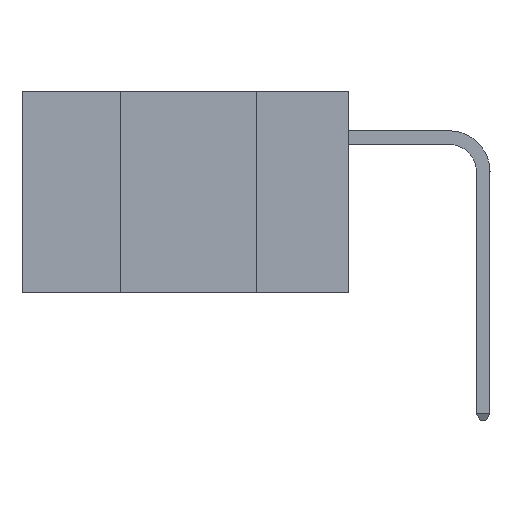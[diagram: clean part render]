
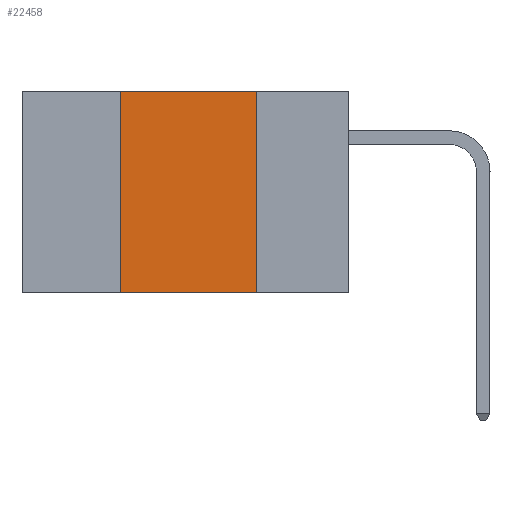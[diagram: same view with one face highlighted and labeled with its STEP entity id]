
A CAD part, left-side view. The second image highlights one B-rep face of the part: STEP entity #22458.
In plain terms, the highlighted planar face has unit normal (-1, 0, 0).
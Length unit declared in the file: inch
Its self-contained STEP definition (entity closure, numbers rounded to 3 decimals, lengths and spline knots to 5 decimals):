
#1540 = VERTEX_POINT ( 'NONE', #36100 ) ;
#1670 = DIRECTION ( 'NONE',  ( 0., 0., -1. ) ) ;
#2449 = PLANE ( 'NONE',  #9147 ) ;
#5805 = DIRECTION ( 'NONE',  ( 0., -1., 0. ) ) ;
#8364 = VECTOR ( 'NONE', #20766, 39.37008 ) ;
#9147 = AXIS2_PLACEMENT_3D ( 'NONE', #11266, #33698, #14107 ) ;
#9754 = CARTESIAN_POINT ( 'NONE',  ( 0., 0.42, 0. ) ) ;
#11266 = CARTESIAN_POINT ( 'NONE',  ( 0., 0.6, 0. ) ) ;
#12080 = DIRECTION ( 'NONE',  ( 0., -1., 0. ) ) ;
#12549 = VECTOR ( 'NONE', #1670, 39.37008 ) ;
#13484 = CARTESIAN_POINT ( 'NONE',  ( 0., 0.17, -0.37 ) ) ;
#14107 = DIRECTION ( 'NONE',  ( 0., 0., -1. ) ) ;
#16509 = VERTEX_POINT ( 'NONE', #13484 ) ;
#17038 = ORIENTED_EDGE ( 'NONE', *, *, #22952, .F. ) ;
#17661 = LINE ( 'NONE', #22747, #28780 ) ;
#18862 = VECTOR ( 'NONE', #12080, 39.37008 ) ;
#20311 = CARTESIAN_POINT ( 'NONE',  ( 0., 0.42, 0. ) ) ;
#20766 = DIRECTION ( 'NONE',  ( 0., 0., 1. ) ) ;
#21460 = VERTEX_POINT ( 'NONE', #26294 ) ;
#21655 = LINE ( 'NONE', #9754, #8364 ) ;
#22458 = ADVANCED_FACE ( 'NONE', ( #29204 ), #2449, .F. ) ;
#22747 = CARTESIAN_POINT ( 'NONE',  ( 0., 0.6, -0.37 ) ) ;
#22952 = EDGE_CURVE ( 'NONE', #27717, #1540, #26403, .T. ) ;
#24914 = EDGE_CURVE ( 'NONE', #1540, #16509, #27965, .T. ) ;
#26294 = CARTESIAN_POINT ( 'NONE',  ( 0., 0.42, -0.37 ) ) ;
#26403 = LINE ( 'NONE', #29009, #18862 ) ;
#27717 = VERTEX_POINT ( 'NONE', #20311 ) ;
#27965 = LINE ( 'NONE', #35552, #12549 ) ;
#28780 = VECTOR ( 'NONE', #5805, 39.37008 ) ;
#29009 = CARTESIAN_POINT ( 'NONE',  ( 0., 0.6, 0. ) ) ;
#29172 = ORIENTED_EDGE ( 'NONE', *, *, #34666, .T. ) ;
#29204 = FACE_OUTER_BOUND ( 'NONE', #31920, .T. ) ;
#31920 = EDGE_LOOP ( 'NONE', ( #34728, #17038, #35727, #29172 ) ) ;
#33698 = DIRECTION ( 'NONE',  ( 1., 0., 0. ) ) ;
#34666 = EDGE_CURVE ( 'NONE', #21460, #16509, #17661, .T. ) ;
#34728 = ORIENTED_EDGE ( 'NONE', *, *, #24914, .F. ) ;
#34883 = EDGE_CURVE ( 'NONE', #21460, #27717, #21655, .T. ) ;
#35552 = CARTESIAN_POINT ( 'NONE',  ( 0., 0.17, 0. ) ) ;
#35727 = ORIENTED_EDGE ( 'NONE', *, *, #34883, .F. ) ;
#36100 = CARTESIAN_POINT ( 'NONE',  ( 0., 0.17, 0. ) ) ;
